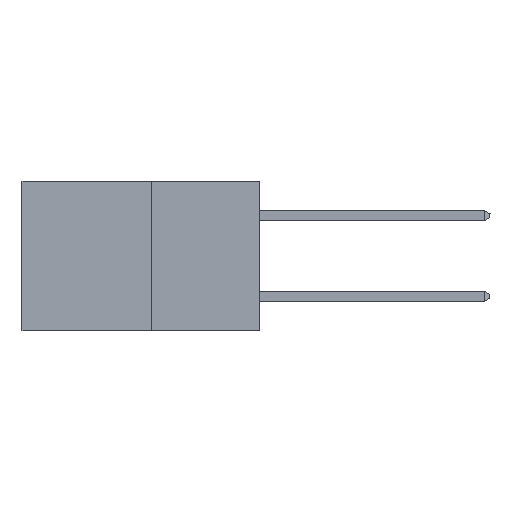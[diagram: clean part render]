
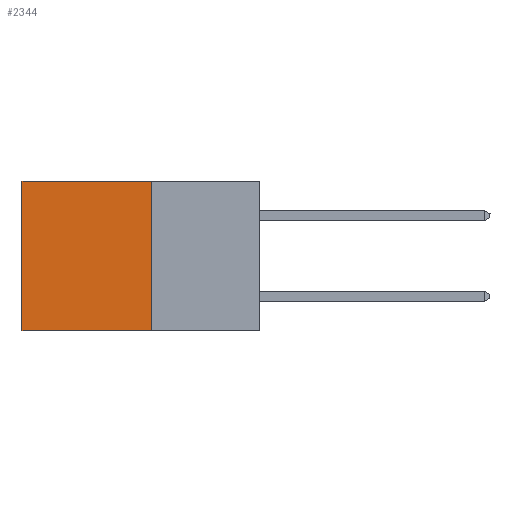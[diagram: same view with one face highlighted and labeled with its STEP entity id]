
A CAD part, left-side view. The second image highlights one B-rep face of the part: STEP entity #2344.
In plain terms, the highlighted planar face has unit normal (-1, 0, 0).
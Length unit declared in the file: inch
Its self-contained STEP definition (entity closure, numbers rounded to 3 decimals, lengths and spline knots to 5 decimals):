
#45 = CARTESIAN_POINT ( 'NONE',  ( 0.277, 0.27, 0. ) ) ;
#101 = CARTESIAN_POINT ( 'NONE',  ( 0.277, 0.27, -0.37 ) ) ;
#494 = AXIS2_PLACEMENT_3D ( 'NONE', #101, #1619, #844 ) ;
#844 = DIRECTION ( 'NONE',  ( 0., 0., -1. ) ) ;
#872 = VECTOR ( 'NONE', #10571, 39.37008 ) ;
#1097 = VERTEX_POINT ( 'NONE', #8930 ) ;
#1176 = CARTESIAN_POINT ( 'NONE',  ( 0.277, 0.27, -0.37 ) ) ;
#1207 = CARTESIAN_POINT ( 'NONE',  ( 0.277, 0.27, -0.37 ) ) ;
#1210 = DIRECTION ( 'NONE',  ( 0., 0., -1. ) ) ;
#1217 = ORIENTED_EDGE ( 'NONE', *, *, #7658, .T. ) ;
#1619 = DIRECTION ( 'NONE',  ( 1., 0., 0. ) ) ;
#1631 = PLANE ( 'NONE',  #494 ) ;
#2023 = VERTEX_POINT ( 'NONE', #4810 ) ;
#2344 = ADVANCED_FACE ( 'NONE', ( #6214 ), #1631, .F. ) ;
#2819 = EDGE_CURVE ( 'NONE', #1097, #10835, #10305, .T. ) ;
#3585 = VECTOR ( 'NONE', #1210, 39.37008 ) ;
#3856 = CARTESIAN_POINT ( 'NONE',  ( 0.277, 0.59, -0.37 ) ) ;
#4218 = EDGE_CURVE ( 'NONE', #2023, #10835, #8529, .T. ) ;
#4810 = CARTESIAN_POINT ( 'NONE',  ( 0.277, 0.27, -0.37 ) ) ;
#6214 = FACE_OUTER_BOUND ( 'NONE', #8889, .T. ) ;
#7512 = DIRECTION ( 'NONE',  ( 0., 0., -1. ) ) ;
#7658 = EDGE_CURVE ( 'NONE', #9802, #1097, #8210, .T. ) ;
#7992 = ORIENTED_EDGE ( 'NONE', *, *, #2819, .T. ) ;
#8210 = LINE ( 'NONE', #8834, #872 ) ;
#8247 = VECTOR ( 'NONE', #8559, 39.37008 ) ;
#8273 = ORIENTED_EDGE ( 'NONE', *, *, #4218, .F. ) ;
#8529 = LINE ( 'NONE', #1207, #8247 ) ;
#8559 = DIRECTION ( 'NONE',  ( 0., 1., 0. ) ) ;
#8834 = CARTESIAN_POINT ( 'NONE',  ( 0.277, 0.27, 0. ) ) ;
#8889 = EDGE_LOOP ( 'NONE', ( #7992, #8273, #10568, #1217 ) ) ;
#8930 = CARTESIAN_POINT ( 'NONE',  ( 0.277, 0.59, 0. ) ) ;
#9442 = EDGE_CURVE ( 'NONE', #9802, #2023, #11016, .T. ) ;
#9802 = VERTEX_POINT ( 'NONE', #45 ) ;
#10039 = VECTOR ( 'NONE', #7512, 39.37008 ) ;
#10305 = LINE ( 'NONE', #3856, #10039 ) ;
#10453 = CARTESIAN_POINT ( 'NONE',  ( 0.277, 0.59, -0.37 ) ) ;
#10568 = ORIENTED_EDGE ( 'NONE', *, *, #9442, .F. ) ;
#10571 = DIRECTION ( 'NONE',  ( 0., 1., 0. ) ) ;
#10835 = VERTEX_POINT ( 'NONE', #10453 ) ;
#11016 = LINE ( 'NONE', #1176, #3585 ) ;
